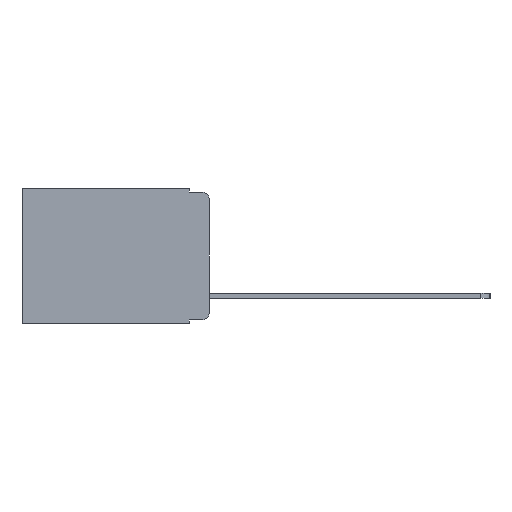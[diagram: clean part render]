
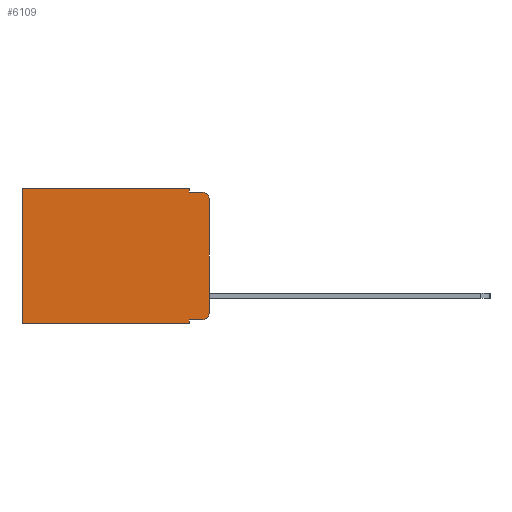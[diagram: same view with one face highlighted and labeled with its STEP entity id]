
A CAD part, left-side view. The second image highlights one B-rep face of the part: STEP entity #6109.
In plain terms, the highlighted planar face has unit normal (-1, 0, 0).
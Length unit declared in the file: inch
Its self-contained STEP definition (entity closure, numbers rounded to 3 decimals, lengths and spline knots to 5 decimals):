
#406 = DIRECTION ( 'NONE',  ( 0., -1., 0. ) ) ;
#743 = CARTESIAN_POINT ( 'NONE',  ( 0.298, 0., -0.313 ) ) ;
#892 = ORIENTED_EDGE ( 'NONE', *, *, #18592, .F. ) ;
#1032 = CARTESIAN_POINT ( 'NONE',  ( 0.298, 0.051, 0. ) ) ;
#1278 = CARTESIAN_POINT ( 'NONE',  ( 0.298, 0.051, -0.333 ) ) ;
#1676 = ORIENTED_EDGE ( 'NONE', *, *, #2406, .F. ) ;
#1724 = DIRECTION ( 'NONE',  ( 0., -1., 0. ) ) ;
#2126 = CARTESIAN_POINT ( 'NONE',  ( 0.298, 0.473, 0. ) ) ;
#2184 = ORIENTED_EDGE ( 'NONE', *, *, #11759, .T. ) ;
#2354 = CIRCLE ( 'NONE', #10902, 0.02 ) ;
#2406 = EDGE_CURVE ( 'NONE', #12209, #13300, #11638, .T. ) ;
#2473 = CARTESIAN_POINT ( 'NONE',  ( 0.298, 0.051, -0.01 ) ) ;
#2509 = LINE ( 'NONE', #10358, #17754 ) ;
#3036 = CARTESIAN_POINT ( 'NONE',  ( 0.298, 0.473, 0. ) ) ;
#3282 = DIRECTION ( 'NONE',  ( 0., 0., -1. ) ) ;
#3372 = CARTESIAN_POINT ( 'NONE',  ( 0.298, 0.473, -0.343 ) ) ;
#3906 = ORIENTED_EDGE ( 'NONE', *, *, #6870, .T. ) ;
#4484 = EDGE_CURVE ( 'NONE', #12136, #13300, #9788, .T. ) ;
#4991 = CARTESIAN_POINT ( 'NONE',  ( 0.298, 0., 0. ) ) ;
#5019 = VERTEX_POINT ( 'NONE', #12669 ) ;
#5148 = CARTESIAN_POINT ( 'NONE',  ( 0.298, 0.02, -0.03 ) ) ;
#5152 = VERTEX_POINT ( 'NONE', #11033 ) ;
#5185 = LINE ( 'NONE', #18236, #9132 ) ;
#5276 = CARTESIAN_POINT ( 'NONE',  ( 0.298, 0., -0.03 ) ) ;
#5418 = CARTESIAN_POINT ( 'NONE',  ( 0.298, 0.02, -0.313 ) ) ;
#5554 = VERTEX_POINT ( 'NONE', #3372 ) ;
#5686 = VECTOR ( 'NONE', #8351, 39.37008 ) ;
#5793 = LINE ( 'NONE', #6649, #9268 ) ;
#6109 = ADVANCED_FACE ( 'NONE', ( #7493 ), #10680, .F. ) ;
#6320 = AXIS2_PLACEMENT_3D ( 'NONE', #7786, #12177, #3282 ) ;
#6471 = CARTESIAN_POINT ( 'NONE',  ( 0.298, 0., 0. ) ) ;
#6639 = VECTOR ( 'NONE', #11912, 39.37008 ) ;
#6649 = CARTESIAN_POINT ( 'NONE',  ( 0.298, 0.051, -0.333 ) ) ;
#6664 = DIRECTION ( 'NONE',  ( 0., 0., -1. ) ) ;
#6870 = EDGE_CURVE ( 'NONE', #14246, #5019, #5793, .T. ) ;
#6934 = DIRECTION ( 'NONE',  ( 0., 0., -1. ) ) ;
#6959 = VERTEX_POINT ( 'NONE', #2126 ) ;
#6963 = ORIENTED_EDGE ( 'NONE', *, *, #7520, .F. ) ;
#7189 = VERTEX_POINT ( 'NONE', #1032 ) ;
#7205 = EDGE_LOOP ( 'NONE', ( #6963, #15641, #1676, #892, #10401, #9033, #17238, #10829, #3906, #2184 ) ) ;
#7493 = FACE_OUTER_BOUND ( 'NONE', #7205, .T. ) ;
#7520 = EDGE_CURVE ( 'NONE', #12136, #18909, #14285, .T. ) ;
#7786 = CARTESIAN_POINT ( 'NONE',  ( 0.298, 0., 0. ) ) ;
#7928 = DIRECTION ( 'NONE',  ( 0., 1., 0. ) ) ;
#8351 = DIRECTION ( 'NONE',  ( 0., 1., 0. ) ) ;
#9033 = ORIENTED_EDGE ( 'NONE', *, *, #15676, .T. ) ;
#9132 = VECTOR ( 'NONE', #9527, 39.37008 ) ;
#9268 = VECTOR ( 'NONE', #406, 39.37008 ) ;
#9527 = DIRECTION ( 'NONE',  ( 0., 0., -1. ) ) ;
#9618 = LINE ( 'NONE', #11190, #5686 ) ;
#9705 = EDGE_CURVE ( 'NONE', #5152, #5554, #9618, .T. ) ;
#9788 = CIRCLE ( 'NONE', #19233, 0.02 ) ;
#9850 = CARTESIAN_POINT ( 'NONE',  ( 0.298, 0.051, -0.01 ) ) ;
#10166 = VECTOR ( 'NONE', #7928, 39.37008 ) ;
#10358 = CARTESIAN_POINT ( 'NONE',  ( 0.298, 0.051, 0. ) ) ;
#10401 = ORIENTED_EDGE ( 'NONE', *, *, #14406, .T. ) ;
#10680 = PLANE ( 'NONE',  #6320 ) ;
#10829 = ORIENTED_EDGE ( 'NONE', *, *, #12768, .F. ) ;
#10902 = AXIS2_PLACEMENT_3D ( 'NONE', #5418, #15672, #6934 ) ;
#11033 = CARTESIAN_POINT ( 'NONE',  ( 0.298, 0.051, -0.343 ) ) ;
#11190 = CARTESIAN_POINT ( 'NONE',  ( 0.298, 0., -0.343 ) ) ;
#11638 = LINE ( 'NONE', #2473, #19358 ) ;
#11759 = EDGE_CURVE ( 'NONE', #5019, #18909, #2354, .T. ) ;
#11912 = DIRECTION ( 'NONE',  ( 0., 0., -1. ) ) ;
#12136 = VERTEX_POINT ( 'NONE', #5276 ) ;
#12177 = DIRECTION ( 'NONE',  ( 1., 0., 0. ) ) ;
#12209 = VERTEX_POINT ( 'NONE', #9850 ) ;
#12669 = CARTESIAN_POINT ( 'NONE',  ( 0.298, 0.02, -0.333 ) ) ;
#12768 = EDGE_CURVE ( 'NONE', #14246, #5152, #5185, .T. ) ;
#13300 = VERTEX_POINT ( 'NONE', #17974 ) ;
#13324 = DIRECTION ( 'NONE',  ( 0., 0., -1. ) ) ;
#14246 = VERTEX_POINT ( 'NONE', #1278 ) ;
#14285 = LINE ( 'NONE', #6471, #14746 ) ;
#14406 = EDGE_CURVE ( 'NONE', #7189, #6959, #18372, .T. ) ;
#14746 = VECTOR ( 'NONE', #16689, 39.37008 ) ;
#15409 = DIRECTION ( 'NONE',  ( -1., 0., 0. ) ) ;
#15641 = ORIENTED_EDGE ( 'NONE', *, *, #4484, .T. ) ;
#15672 = DIRECTION ( 'NONE',  ( -1., 0., 0. ) ) ;
#15676 = EDGE_CURVE ( 'NONE', #6959, #5554, #17826, .T. ) ;
#16689 = DIRECTION ( 'NONE',  ( 0., 0., -1. ) ) ;
#17238 = ORIENTED_EDGE ( 'NONE', *, *, #9705, .F. ) ;
#17754 = VECTOR ( 'NONE', #13324, 39.37008 ) ;
#17826 = LINE ( 'NONE', #3036, #6639 ) ;
#17974 = CARTESIAN_POINT ( 'NONE',  ( 0.298, 0.02, -0.01 ) ) ;
#18236 = CARTESIAN_POINT ( 'NONE',  ( 0.298, 0.051, 0. ) ) ;
#18372 = LINE ( 'NONE', #4991, #10166 ) ;
#18592 = EDGE_CURVE ( 'NONE', #7189, #12209, #2509, .T. ) ;
#18909 = VERTEX_POINT ( 'NONE', #743 ) ;
#19233 = AXIS2_PLACEMENT_3D ( 'NONE', #5148, #15409, #6664 ) ;
#19358 = VECTOR ( 'NONE', #1724, 39.37008 ) ;
